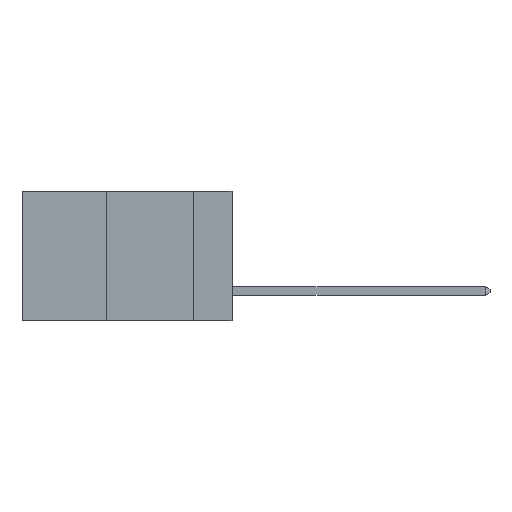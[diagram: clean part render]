
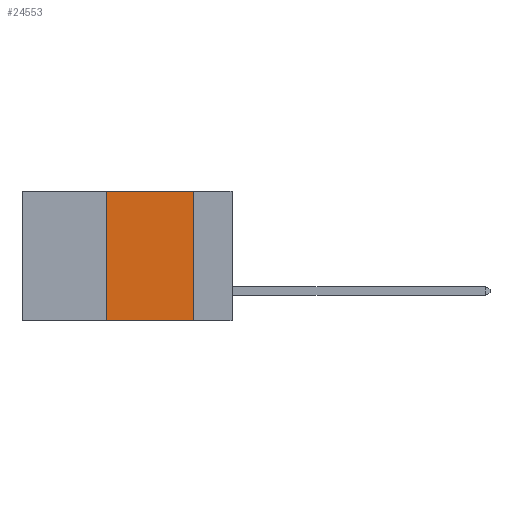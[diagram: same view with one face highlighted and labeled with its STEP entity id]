
A CAD part, left-side view. The second image highlights one B-rep face of the part: STEP entity #24553.
In plain terms, the highlighted planar face has unit normal (-1, 0, 0).
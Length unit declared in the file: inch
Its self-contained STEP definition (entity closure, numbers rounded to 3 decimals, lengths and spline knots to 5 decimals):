
#233 = CARTESIAN_POINT ( 'NONE',  ( 0., 0.36, -0.37 ) ) ;
#288 = CARTESIAN_POINT ( 'NONE',  ( 0., 0.6, -0.37 ) ) ;
#1588 = AXIS2_PLACEMENT_3D ( 'NONE', #28332, #15346, #1888 ) ;
#1888 = DIRECTION ( 'NONE',  ( 0., 0., -1. ) ) ;
#2346 = VERTEX_POINT ( 'NONE', #26616 ) ;
#3269 = VECTOR ( 'NONE', #9614, 39.37008 ) ;
#3470 = VERTEX_POINT ( 'NONE', #233 ) ;
#6032 = LINE ( 'NONE', #6896, #22202 ) ;
#6165 = ORIENTED_EDGE ( 'NONE', *, *, #6174, .F. ) ;
#6174 = EDGE_CURVE ( 'NONE', #3470, #28545, #26490, .T. ) ;
#6881 = ORIENTED_EDGE ( 'NONE', *, *, #12704, .T. ) ;
#6896 = CARTESIAN_POINT ( 'NONE',  ( 0., 0.11, 0. ) ) ;
#7243 = DIRECTION ( 'NONE',  ( 0., 0., 1. ) ) ;
#7730 = EDGE_CURVE ( 'NONE', #28545, #2346, #15855, .T. ) ;
#9272 = FACE_OUTER_BOUND ( 'NONE', #16661, .T. ) ;
#9520 = DIRECTION ( 'NONE',  ( 0., -1., 0. ) ) ;
#9614 = DIRECTION ( 'NONE',  ( 0., -1., 0. ) ) ;
#10944 = PLANE ( 'NONE',  #1588 ) ;
#12704 = EDGE_CURVE ( 'NONE', #3470, #17033, #16224, .T. ) ;
#14012 = CARTESIAN_POINT ( 'NONE',  ( 0., 0.6, 0. ) ) ;
#15346 = DIRECTION ( 'NONE',  ( 1., 0., 0. ) ) ;
#15855 = LINE ( 'NONE', #14012, #3269 ) ;
#16224 = LINE ( 'NONE', #288, #23357 ) ;
#16661 = EDGE_LOOP ( 'NONE', ( #27409, #23010, #6165, #6881 ) ) ;
#17033 = VERTEX_POINT ( 'NONE', #25080 ) ;
#20697 = VECTOR ( 'NONE', #7243, 39.37008 ) ;
#22202 = VECTOR ( 'NONE', #26617, 39.37008 ) ;
#22573 = CARTESIAN_POINT ( 'NONE',  ( 0., 0.36, 0. ) ) ;
#23010 = ORIENTED_EDGE ( 'NONE', *, *, #7730, .F. ) ;
#23357 = VECTOR ( 'NONE', #9520, 39.37008 ) ;
#24553 = ADVANCED_FACE ( 'NONE', ( #9272 ), #10944, .F. ) ;
#24649 = CARTESIAN_POINT ( 'NONE',  ( 0., 0.36, 0. ) ) ;
#25080 = CARTESIAN_POINT ( 'NONE',  ( 0., 0.11, -0.37 ) ) ;
#25318 = EDGE_CURVE ( 'NONE', #2346, #17033, #6032, .T. ) ;
#26490 = LINE ( 'NONE', #22573, #20697 ) ;
#26616 = CARTESIAN_POINT ( 'NONE',  ( 0., 0.11, 0. ) ) ;
#26617 = DIRECTION ( 'NONE',  ( 0., 0., -1. ) ) ;
#27409 = ORIENTED_EDGE ( 'NONE', *, *, #25318, .F. ) ;
#28332 = CARTESIAN_POINT ( 'NONE',  ( 0., 0.6, 0. ) ) ;
#28545 = VERTEX_POINT ( 'NONE', #24649 ) ;
